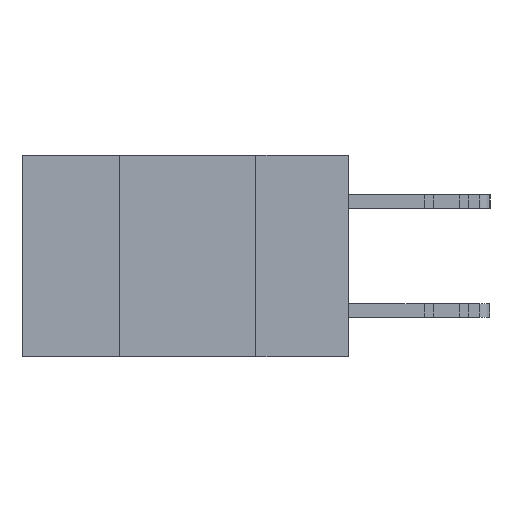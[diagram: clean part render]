
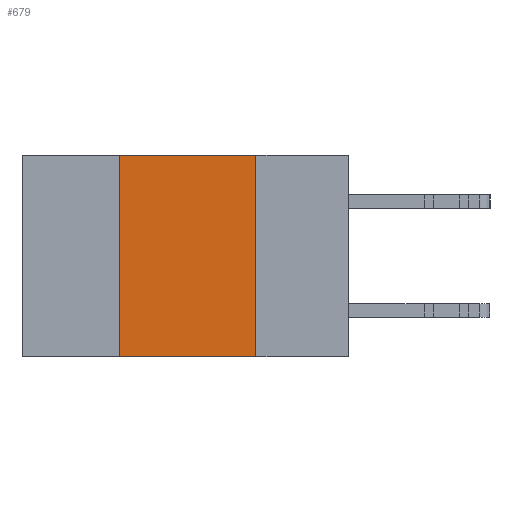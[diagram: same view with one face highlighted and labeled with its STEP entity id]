
A CAD part, left-side view. The second image highlights one B-rep face of the part: STEP entity #679.
In plain terms, the highlighted planar face has unit normal (-1, 0, 0).
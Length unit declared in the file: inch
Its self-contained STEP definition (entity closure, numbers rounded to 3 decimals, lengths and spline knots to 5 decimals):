
#679 = ADVANCED_FACE ( 'NONE', ( #2569 ), #19805, .F. ) ;
#1268 = CARTESIAN_POINT ( 'NONE',  ( 0., 0.6, 0. ) ) ;
#1565 = VERTEX_POINT ( 'NONE', #15587 ) ;
#2447 = CARTESIAN_POINT ( 'NONE',  ( 0., 0.6, 0. ) ) ;
#2569 = FACE_OUTER_BOUND ( 'NONE', #7942, .T. ) ;
#3212 = DIRECTION ( 'NONE',  ( 0., -1., 0. ) ) ;
#3450 = VERTEX_POINT ( 'NONE', #4513 ) ;
#4009 = CARTESIAN_POINT ( 'NONE',  ( 0., 0.42, -0.37 ) ) ;
#4513 = CARTESIAN_POINT ( 'NONE',  ( 0., 0.17, -0.37 ) ) ;
#5001 = ORIENTED_EDGE ( 'NONE', *, *, #8363, .F. ) ;
#6167 = DIRECTION ( 'NONE',  ( 0., -1., 0. ) ) ;
#7942 = EDGE_LOOP ( 'NONE', ( #5001, #22332, #10389, #17616 ) ) ;
#8305 = DIRECTION ( 'NONE',  ( 1., 0., 0. ) ) ;
#8363 = EDGE_CURVE ( 'NONE', #1565, #3450, #24193, .T. ) ;
#8873 = CARTESIAN_POINT ( 'NONE',  ( 0., 0.17, -0.37 ) ) ;
#9525 = EDGE_CURVE ( 'NONE', #17360, #1565, #15249, .T. ) ;
#9605 = LINE ( 'NONE', #4009, #22412 ) ;
#9984 = DIRECTION ( 'NONE',  ( 0., 0., 1. ) ) ;
#10389 = ORIENTED_EDGE ( 'NONE', *, *, #21778, .F. ) ;
#10566 = VERTEX_POINT ( 'NONE', #15076 ) ;
#10614 = AXIS2_PLACEMENT_3D ( 'NONE', #2447, #8305, #16268 ) ;
#13836 = EDGE_CURVE ( 'NONE', #10566, #3450, #14025, .T. ) ;
#14025 = LINE ( 'NONE', #18168, #23432 ) ;
#15076 = CARTESIAN_POINT ( 'NONE',  ( 0., 0.42, -0.37 ) ) ;
#15249 = LINE ( 'NONE', #1268, #20010 ) ;
#15587 = CARTESIAN_POINT ( 'NONE',  ( 0., 0.17, 0. ) ) ;
#16268 = DIRECTION ( 'NONE',  ( 0., 0., -1. ) ) ;
#17360 = VERTEX_POINT ( 'NONE', #21101 ) ;
#17616 = ORIENTED_EDGE ( 'NONE', *, *, #13836, .T. ) ;
#18168 = CARTESIAN_POINT ( 'NONE',  ( 0., 0.6, -0.37 ) ) ;
#18588 = DIRECTION ( 'NONE',  ( 0., 0., -1. ) ) ;
#19805 = PLANE ( 'NONE',  #10614 ) ;
#20010 = VECTOR ( 'NONE', #3212, 39.37008 ) ;
#20847 = VECTOR ( 'NONE', #18588, 39.37008 ) ;
#21101 = CARTESIAN_POINT ( 'NONE',  ( 0., 0.42, 0. ) ) ;
#21778 = EDGE_CURVE ( 'NONE', #10566, #17360, #9605, .T. ) ;
#22332 = ORIENTED_EDGE ( 'NONE', *, *, #9525, .F. ) ;
#22412 = VECTOR ( 'NONE', #9984, 39.37008 ) ;
#23432 = VECTOR ( 'NONE', #6167, 39.37008 ) ;
#24193 = LINE ( 'NONE', #8873, #20847 ) ;
